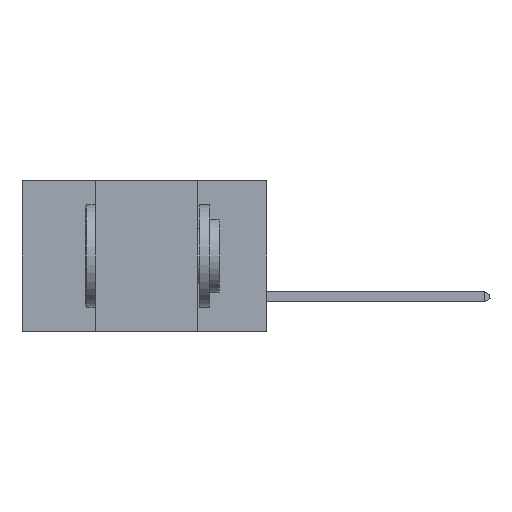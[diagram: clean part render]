
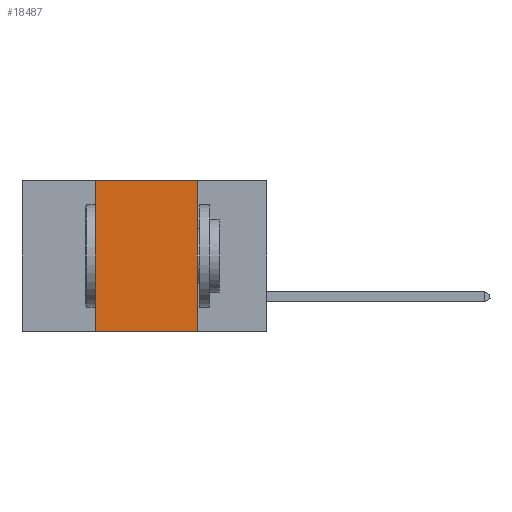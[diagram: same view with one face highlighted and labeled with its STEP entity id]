
A CAD part, left-side view. The second image highlights one B-rep face of the part: STEP entity #18487.
In plain terms, the highlighted planar face has unit normal (-1, 0, 0).
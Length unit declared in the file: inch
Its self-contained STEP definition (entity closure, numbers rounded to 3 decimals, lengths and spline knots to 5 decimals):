
#2106 = EDGE_CURVE ( 'NONE', #2979, #10681, #15442, .T. ) ;
#2471 = CARTESIAN_POINT ( 'NONE',  ( 0., 0.17, -0.37 ) ) ;
#2979 = VERTEX_POINT ( 'NONE', #6530 ) ;
#3012 = LINE ( 'NONE', #10095, #33371 ) ;
#6530 = CARTESIAN_POINT ( 'NONE',  ( 0., 0.42, 0. ) ) ;
#7077 = LINE ( 'NONE', #30617, #33207 ) ;
#7372 = FACE_OUTER_BOUND ( 'NONE', #41180, .T. ) ;
#10095 = CARTESIAN_POINT ( 'NONE',  ( 0., 0.42, 0. ) ) ;
#10681 = VERTEX_POINT ( 'NONE', #26853 ) ;
#10930 = VERTEX_POINT ( 'NONE', #43925 ) ;
#11825 = DIRECTION ( 'NONE',  ( 0., -1., 0. ) ) ;
#12154 = EDGE_CURVE ( 'NONE', #10930, #18340, #34958, .T. ) ;
#13495 = CARTESIAN_POINT ( 'NONE',  ( 0., 0.6, 0. ) ) ;
#14106 = DIRECTION ( 'NONE',  ( 0., 0., -1. ) ) ;
#15070 = CARTESIAN_POINT ( 'NONE',  ( 0., 0.6, -0.37 ) ) ;
#15442 = LINE ( 'NONE', #32724, #26112 ) ;
#15808 = VECTOR ( 'NONE', #11825, 39.37008 ) ;
#16169 = EDGE_CURVE ( 'NONE', #10681, #18340, #7077, .T. ) ;
#18340 = VERTEX_POINT ( 'NONE', #2471 ) ;
#18487 = ADVANCED_FACE ( 'NONE', ( #7372 ), #19847, .F. ) ;
#19847 = PLANE ( 'NONE',  #23880 ) ;
#20133 = DIRECTION ( 'NONE',  ( 1., 0., 0. ) ) ;
#22901 = ORIENTED_EDGE ( 'NONE', *, *, #2106, .F. ) ;
#23275 = DIRECTION ( 'NONE',  ( 0., 0., -1. ) ) ;
#23303 = ORIENTED_EDGE ( 'NONE', *, *, #12154, .T. ) ;
#23880 = AXIS2_PLACEMENT_3D ( 'NONE', #13495, #20133, #23275 ) ;
#25896 = EDGE_CURVE ( 'NONE', #10930, #2979, #3012, .T. ) ;
#26112 = VECTOR ( 'NONE', #38994, 39.37008 ) ;
#26197 = ORIENTED_EDGE ( 'NONE', *, *, #16169, .F. ) ;
#26853 = CARTESIAN_POINT ( 'NONE',  ( 0., 0.17, 0. ) ) ;
#26907 = DIRECTION ( 'NONE',  ( 0., 0., 1. ) ) ;
#30617 = CARTESIAN_POINT ( 'NONE',  ( 0., 0.17, 0. ) ) ;
#32386 = ORIENTED_EDGE ( 'NONE', *, *, #25896, .F. ) ;
#32724 = CARTESIAN_POINT ( 'NONE',  ( 0., 0.6, 0. ) ) ;
#33207 = VECTOR ( 'NONE', #14106, 39.37008 ) ;
#33371 = VECTOR ( 'NONE', #26907, 39.37008 ) ;
#34958 = LINE ( 'NONE', #15070, #15808 ) ;
#38994 = DIRECTION ( 'NONE',  ( 0., -1., 0. ) ) ;
#41180 = EDGE_LOOP ( 'NONE', ( #26197, #22901, #32386, #23303 ) ) ;
#43925 = CARTESIAN_POINT ( 'NONE',  ( 0., 0.42, -0.37 ) ) ;
